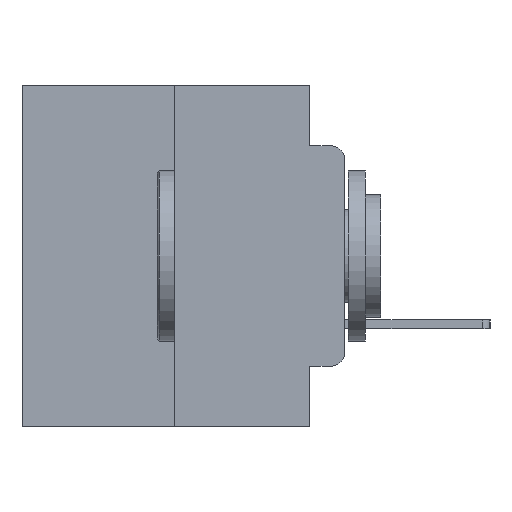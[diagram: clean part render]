
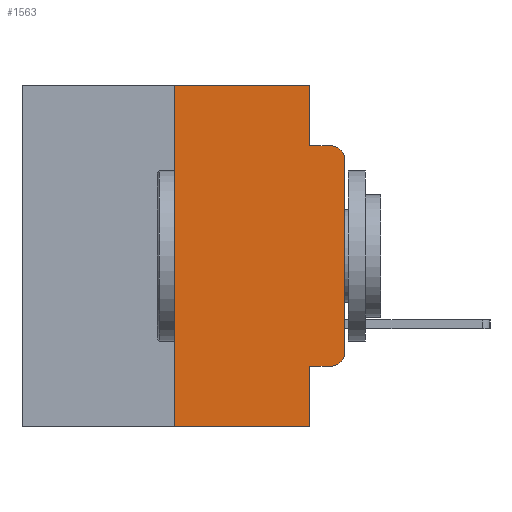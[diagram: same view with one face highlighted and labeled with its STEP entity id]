
A CAD part, left-side view. The second image highlights one B-rep face of the part: STEP entity #1563.
In plain terms, the highlighted planar face has unit normal (-1, 0, 0).
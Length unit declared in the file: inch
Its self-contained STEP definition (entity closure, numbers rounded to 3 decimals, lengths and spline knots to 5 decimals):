
#379 = EDGE_LOOP ( 'NONE', ( #6943, #12989, #24297, #3271, #14902, #26169, #5977, #16794, #12704, #18057 ) ) ;
#383 = CARTESIAN_POINT ( 'NONE',  ( 0., 0.051, -0.4115 ) ) ;
#1084 = CARTESIAN_POINT ( 'NONE',  ( 0., 0.051, -0.0885 ) ) ;
#1563 = ADVANCED_FACE ( 'NONE', ( #5929 ), #16370, .F. ) ;
#1603 = VERTEX_POINT ( 'NONE', #8543 ) ;
#2000 = EDGE_CURVE ( 'NONE', #26468, #1603, #26105, .T. ) ;
#2611 = DIRECTION ( 'NONE',  ( 0., -1., 0. ) ) ;
#3086 = VERTEX_POINT ( 'NONE', #18380 ) ;
#3271 = ORIENTED_EDGE ( 'NONE', *, *, #17431, .F. ) ;
#4233 = EDGE_CURVE ( 'NONE', #23590, #11624, #25261, .T. ) ;
#4378 = VECTOR ( 'NONE', #14888, 39.37008 ) ;
#4586 = VECTOR ( 'NONE', #2611, 39.37008 ) ;
#4595 = VECTOR ( 'NONE', #14716, 39.37008 ) ;
#4665 = CARTESIAN_POINT ( 'NONE',  ( 0., 0.051, 0. ) ) ;
#4794 = CIRCLE ( 'NONE', #9696, 0.02 ) ;
#5159 = CIRCLE ( 'NONE', #19810, 0.02 ) ;
#5260 = LINE ( 'NONE', #11034, #4586 ) ;
#5929 = FACE_OUTER_BOUND ( 'NONE', #379, .T. ) ;
#5977 = ORIENTED_EDGE ( 'NONE', *, *, #20801, .T. ) ;
#6242 = DIRECTION ( 'NONE',  ( 1., 0., 0. ) ) ;
#6367 = VECTOR ( 'NONE', #16891, 39.37008 ) ;
#6720 = CARTESIAN_POINT ( 'NONE',  ( 0., 0.25, 0. ) ) ;
#6943 = ORIENTED_EDGE ( 'NONE', *, *, #2000, .T. ) ;
#7004 = LINE ( 'NONE', #10838, #6367 ) ;
#7188 = AXIS2_PLACEMENT_3D ( 'NONE', #22356, #6242, #20425 ) ;
#8457 = EDGE_CURVE ( 'NONE', #1603, #3086, #4794, .T. ) ;
#8543 = CARTESIAN_POINT ( 'NONE',  ( 0., 0., -0.1085 ) ) ;
#8817 = VERTEX_POINT ( 'NONE', #18700 ) ;
#8842 = CARTESIAN_POINT ( 'NONE',  ( 0., 0.02, -0.4115 ) ) ;
#9696 = AXIS2_PLACEMENT_3D ( 'NONE', #11067, #25058, #13071 ) ;
#9942 = EDGE_CURVE ( 'NONE', #16800, #26468, #5159, .T. ) ;
#10772 = VECTOR ( 'NONE', #14141, 39.37008 ) ;
#10790 = LINE ( 'NONE', #14629, #4595 ) ;
#10838 = CARTESIAN_POINT ( 'NONE',  ( 0., 0.051, 0. ) ) ;
#11034 = CARTESIAN_POINT ( 'NONE',  ( 0., 0.473, 0. ) ) ;
#11067 = CARTESIAN_POINT ( 'NONE',  ( 0., 0.02, -0.1085 ) ) ;
#11470 = DIRECTION ( 'NONE',  ( 0., -1., 0. ) ) ;
#11624 = VERTEX_POINT ( 'NONE', #14957 ) ;
#11631 = CARTESIAN_POINT ( 'NONE',  ( 0., 0.02, -0.3915 ) ) ;
#11928 = CARTESIAN_POINT ( 'NONE',  ( 0., 0.473, -0.5 ) ) ;
#12029 = VECTOR ( 'NONE', #22894, 39.37008 ) ;
#12370 = CARTESIAN_POINT ( 'NONE',  ( 0., 0.25, -0.5 ) ) ;
#12704 = ORIENTED_EDGE ( 'NONE', *, *, #25650, .T. ) ;
#12989 = ORIENTED_EDGE ( 'NONE', *, *, #8457, .T. ) ;
#13071 = DIRECTION ( 'NONE',  ( 0., 0., -1. ) ) ;
#13639 = DIRECTION ( 'NONE',  ( 0., 0., -1. ) ) ;
#13942 = DIRECTION ( 'NONE',  ( 0., -1., 0. ) ) ;
#14141 = DIRECTION ( 'NONE',  ( 0., 0., 1. ) ) ;
#14249 = LINE ( 'NONE', #11928, #24270 ) ;
#14259 = VECTOR ( 'NONE', #11470, 39.37008 ) ;
#14629 = CARTESIAN_POINT ( 'NONE',  ( 0., 0.051, -0.4115 ) ) ;
#14716 = DIRECTION ( 'NONE',  ( 0., -1., 0. ) ) ;
#14888 = DIRECTION ( 'NONE',  ( 0., 0., -1. ) ) ;
#14902 = ORIENTED_EDGE ( 'NONE', *, *, #21130, .F. ) ;
#14957 = CARTESIAN_POINT ( 'NONE',  ( 0., 0.051, -0.5 ) ) ;
#15595 = CARTESIAN_POINT ( 'NONE',  ( 0., 0.051, 0. ) ) ;
#16370 = PLANE ( 'NONE',  #7188 ) ;
#16582 = VERTEX_POINT ( 'NONE', #22642 ) ;
#16794 = ORIENTED_EDGE ( 'NONE', *, *, #4233, .F. ) ;
#16800 = VERTEX_POINT ( 'NONE', #8842 ) ;
#16891 = DIRECTION ( 'NONE',  ( 0., 0., -1. ) ) ;
#17373 = LINE ( 'NONE', #6720, #12029 ) ;
#17431 = EDGE_CURVE ( 'NONE', #23083, #8817, #7004, .T. ) ;
#18057 = ORIENTED_EDGE ( 'NONE', *, *, #9942, .T. ) ;
#18380 = CARTESIAN_POINT ( 'NONE',  ( 0., 0.02, -0.0885 ) ) ;
#18700 = CARTESIAN_POINT ( 'NONE',  ( 0., 0.051, -0.0885 ) ) ;
#19810 = AXIS2_PLACEMENT_3D ( 'NONE', #11631, #25632, #13639 ) ;
#20425 = DIRECTION ( 'NONE',  ( 0., 0., -1. ) ) ;
#20801 = EDGE_CURVE ( 'NONE', #24924, #11624, #14249, .T. ) ;
#21088 = EDGE_CURVE ( 'NONE', #24924, #16582, #17373, .T. ) ;
#21130 = EDGE_CURVE ( 'NONE', #16582, #23083, #5260, .T. ) ;
#22356 = CARTESIAN_POINT ( 'NONE',  ( 0., 0.473, 0. ) ) ;
#22642 = CARTESIAN_POINT ( 'NONE',  ( 0., 0.25, 0. ) ) ;
#22894 = DIRECTION ( 'NONE',  ( 0., 0., 1. ) ) ;
#23083 = VERTEX_POINT ( 'NONE', #15595 ) ;
#23590 = VERTEX_POINT ( 'NONE', #383 ) ;
#24270 = VECTOR ( 'NONE', #13942, 39.37008 ) ;
#24297 = ORIENTED_EDGE ( 'NONE', *, *, #25245, .F. ) ;
#24330 = CARTESIAN_POINT ( 'NONE',  ( 0., 0., -0.3915 ) ) ;
#24877 = LINE ( 'NONE', #1084, #14259 ) ;
#24924 = VERTEX_POINT ( 'NONE', #12370 ) ;
#25058 = DIRECTION ( 'NONE',  ( -1., 0., 0. ) ) ;
#25245 = EDGE_CURVE ( 'NONE', #8817, #3086, #24877, .T. ) ;
#25261 = LINE ( 'NONE', #4665, #4378 ) ;
#25632 = DIRECTION ( 'NONE',  ( -1., 0., 0. ) ) ;
#25650 = EDGE_CURVE ( 'NONE', #23590, #16800, #10790, .T. ) ;
#26105 = LINE ( 'NONE', #26121, #10772 ) ;
#26121 = CARTESIAN_POINT ( 'NONE',  ( 0., 0., 0. ) ) ;
#26169 = ORIENTED_EDGE ( 'NONE', *, *, #21088, .F. ) ;
#26468 = VERTEX_POINT ( 'NONE', #24330 ) ;
